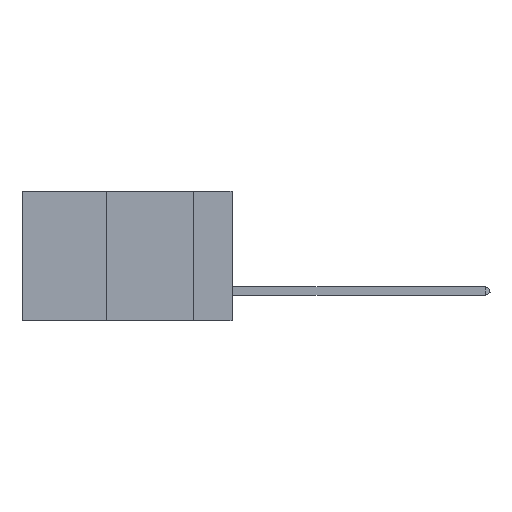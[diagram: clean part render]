
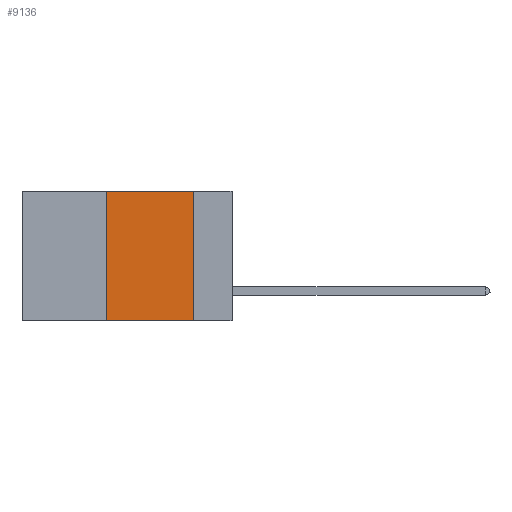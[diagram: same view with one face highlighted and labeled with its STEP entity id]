
A CAD part, left-side view. The second image highlights one B-rep face of the part: STEP entity #9136.
In plain terms, the highlighted planar face has unit normal (-1, 0, 0).
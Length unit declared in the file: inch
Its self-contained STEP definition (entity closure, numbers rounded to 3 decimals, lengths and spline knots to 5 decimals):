
#717 = DIRECTION ( 'NONE',  ( 0., 0., -1. ) ) ;
#2036 = AXIS2_PLACEMENT_3D ( 'NONE', #26707, #22616, #7491 ) ;
#3532 = CARTESIAN_POINT ( 'NONE',  ( 0., 0.36, 0. ) ) ;
#5567 = EDGE_CURVE ( 'NONE', #12565, #7790, #15849, .T. ) ;
#6548 = EDGE_CURVE ( 'NONE', #12565, #16705, #21385, .T. ) ;
#6629 = ORIENTED_EDGE ( 'NONE', *, *, #24908, .F. ) ;
#6677 = VERTEX_POINT ( 'NONE', #20969 ) ;
#7491 = DIRECTION ( 'NONE',  ( 0., 0., -1. ) ) ;
#7790 = VERTEX_POINT ( 'NONE', #3532 ) ;
#8369 = DIRECTION ( 'NONE',  ( 0., 0., 1. ) ) ;
#9136 = ADVANCED_FACE ( 'NONE', ( #10802 ), #14107, .F. ) ;
#10802 = FACE_OUTER_BOUND ( 'NONE', #19189, .T. ) ;
#12565 = VERTEX_POINT ( 'NONE', #18296 ) ;
#12820 = DIRECTION ( 'NONE',  ( 0., -1., 0. ) ) ;
#14107 = PLANE ( 'NONE',  #2036 ) ;
#14257 = VECTOR ( 'NONE', #12820, 39.37008 ) ;
#14370 = ORIENTED_EDGE ( 'NONE', *, *, #6548, .T. ) ;
#15849 = LINE ( 'NONE', #21053, #17509 ) ;
#16705 = VERTEX_POINT ( 'NONE', #24788 ) ;
#17509 = VECTOR ( 'NONE', #8369, 39.37008 ) ;
#18185 = VECTOR ( 'NONE', #717, 39.37008 ) ;
#18189 = ORIENTED_EDGE ( 'NONE', *, *, #5567, .F. ) ;
#18296 = CARTESIAN_POINT ( 'NONE',  ( 0., 0.36, -0.37 ) ) ;
#19189 = EDGE_LOOP ( 'NONE', ( #6629, #26375, #18189, #14370 ) ) ;
#19321 = CARTESIAN_POINT ( 'NONE',  ( 0., 0.6, 0. ) ) ;
#19476 = CARTESIAN_POINT ( 'NONE',  ( 0., 0.11, 0. ) ) ;
#20876 = CARTESIAN_POINT ( 'NONE',  ( 0., 0.6, -0.37 ) ) ;
#20969 = CARTESIAN_POINT ( 'NONE',  ( 0., 0.11, 0. ) ) ;
#21053 = CARTESIAN_POINT ( 'NONE',  ( 0., 0.36, 0. ) ) ;
#21385 = LINE ( 'NONE', #20876, #26732 ) ;
#21579 = LINE ( 'NONE', #19321, #14257 ) ;
#22616 = DIRECTION ( 'NONE',  ( 1., 0., 0. ) ) ;
#23561 = EDGE_CURVE ( 'NONE', #7790, #6677, #21579, .T. ) ;
#24788 = CARTESIAN_POINT ( 'NONE',  ( 0., 0.11, -0.37 ) ) ;
#24908 = EDGE_CURVE ( 'NONE', #6677, #16705, #26088, .T. ) ;
#25741 = DIRECTION ( 'NONE',  ( 0., -1., 0. ) ) ;
#26088 = LINE ( 'NONE', #19476, #18185 ) ;
#26375 = ORIENTED_EDGE ( 'NONE', *, *, #23561, .F. ) ;
#26707 = CARTESIAN_POINT ( 'NONE',  ( 0., 0.6, 0. ) ) ;
#26732 = VECTOR ( 'NONE', #25741, 39.37008 ) ;
